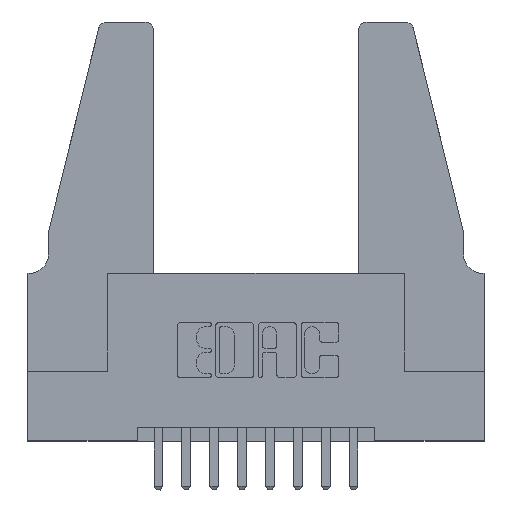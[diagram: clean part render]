
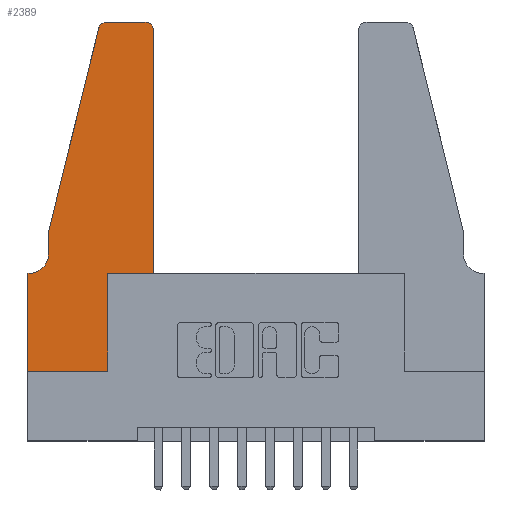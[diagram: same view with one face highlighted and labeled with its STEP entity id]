
A CAD part, top view. The second image highlights one B-rep face of the part: STEP entity #2389.
In plain terms, the highlighted planar face has unit normal (0, 0, 1).
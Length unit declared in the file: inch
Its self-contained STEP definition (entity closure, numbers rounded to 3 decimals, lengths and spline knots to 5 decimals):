
#106 = VECTOR ( 'NONE', #6121, 39.37008 ) ;
#154 = LINE ( 'NONE', #10776, #2517 ) ;
#213 = LINE ( 'NONE', #10357, #3708 ) ;
#300 = CARTESIAN_POINT ( 'NONE',  ( 0.2605, 1.25, 0.37 ) ) ;
#664 = CARTESIAN_POINT ( 'NONE',  ( 0.0755, 0.5, 0.37 ) ) ;
#752 = CARTESIAN_POINT ( 'NONE',  ( 0.4205, 1.25, 0.37 ) ) ;
#1054 = ORIENTED_EDGE ( 'NONE', *, *, #2279, .T. ) ;
#1104 = CARTESIAN_POINT ( 'NONE',  ( 0.4505, 0.35, 0.37 ) ) ;
#1106 = FACE_OUTER_BOUND ( 'NONE', #12802, .T. ) ;
#1151 = ORIENTED_EDGE ( 'NONE', *, *, #7152, .T. ) ;
#1360 = VERTEX_POINT ( 'NONE', #5652 ) ;
#1537 = CARTESIAN_POINT ( 'NONE',  ( 0.4505, 0.35, 0.37 ) ) ;
#1848 = EDGE_CURVE ( 'NONE', #4056, #9533, #4772, .T. ) ;
#1996 = VERTEX_POINT ( 'NONE', #5301 ) ;
#2011 = ORIENTED_EDGE ( 'NONE', *, *, #8331, .T. ) ;
#2022 = CARTESIAN_POINT ( 'NONE',  ( 0.0055, 0.35, 0.37 ) ) ;
#2279 = EDGE_CURVE ( 'NONE', #9148, #5558, #9391, .T. ) ;
#2302 = DIRECTION ( 'NONE',  ( -1., 0., 0. ) ) ;
#2389 = ADVANCED_FACE ( 'NONE', ( #1106 ), #4927, .T. ) ;
#2517 = VECTOR ( 'NONE', #8814, 39.37008 ) ;
#2630 = LINE ( 'NONE', #300, #12486 ) ;
#2672 = VERTEX_POINT ( 'NONE', #1537 ) ;
#2903 = VECTOR ( 'NONE', #11916, 39.37008 ) ;
#3019 = CARTESIAN_POINT ( 'NONE',  ( 0.2865, 0.35, 0.37 ) ) ;
#3112 = ORIENTED_EDGE ( 'NONE', *, *, #9531, .T. ) ;
#3143 = DIRECTION ( 'NONE',  ( 0., 1., 0. ) ) ;
#3332 = VECTOR ( 'NONE', #7789, 39.37008 ) ;
#3708 = VECTOR ( 'NONE', #5157, 39.37008 ) ;
#3750 = LINE ( 'NONE', #1104, #9966 ) ;
#4056 = VERTEX_POINT ( 'NONE', #5022 ) ;
#4112 = DIRECTION ( 'NONE',  ( 0., 0., 1. ) ) ;
#4241 = VERTEX_POINT ( 'NONE', #9990 ) ;
#4388 = CARTESIAN_POINT ( 'NONE',  ( 0.0755, 0.35, 0.37 ) ) ;
#4525 = CARTESIAN_POINT ( 'NONE',  ( 0.284, 1.22, 0.37 ) ) ;
#4729 = VECTOR ( 'NONE', #2302, 39.37008 ) ;
#4732 = CARTESIAN_POINT ( 'NONE',  ( 0.0755, 0.5, 0.37 ) ) ;
#4772 = LINE ( 'NONE', #3019, #6977 ) ;
#4849 = EDGE_CURVE ( 'NONE', #6688, #4056, #9325, .T. ) ;
#4927 = PLANE ( 'NONE',  #9823 ) ;
#5022 = CARTESIAN_POINT ( 'NONE',  ( 0.2865, 0., 0.37 ) ) ;
#5157 = DIRECTION ( 'NONE',  ( 1., 0., 0. ) ) ;
#5158 = EDGE_CURVE ( 'NONE', #1996, #4241, #12277, .T. ) ;
#5301 = CARTESIAN_POINT ( 'NONE',  ( 0.284, 1.25, 0.37 ) ) ;
#5397 = VERTEX_POINT ( 'NONE', #2022 ) ;
#5548 = DIRECTION ( 'NONE',  ( 0., 0., 1. ) ) ;
#5558 = VERTEX_POINT ( 'NONE', #7527 ) ;
#5594 = LINE ( 'NONE', #664, #2903 ) ;
#5596 = DIRECTION ( 'NONE',  ( 1., 0., 0. ) ) ;
#5619 = ORIENTED_EDGE ( 'NONE', *, *, #10081, .T. ) ;
#5630 = VERTEX_POINT ( 'NONE', #7299 ) ;
#5652 = CARTESIAN_POINT ( 'NONE',  ( 0.4505, 1.22, 0.37 ) ) ;
#5856 = ORIENTED_EDGE ( 'NONE', *, *, #10337, .T. ) ;
#5931 = ORIENTED_EDGE ( 'NONE', *, *, #8153, .T. ) ;
#6121 = DIRECTION ( 'NONE',  ( 1., 0., 0. ) ) ;
#6528 = ORIENTED_EDGE ( 'NONE', *, *, #12470, .T. ) ;
#6688 = VERTEX_POINT ( 'NONE', #8548 ) ;
#6740 = ORIENTED_EDGE ( 'NONE', *, *, #4849, .T. ) ;
#6977 = VECTOR ( 'NONE', #12147, 39.37008 ) ;
#6981 = CARTESIAN_POINT ( 'NONE',  ( 0., 0.35, 0.37 ) ) ;
#7152 = EDGE_CURVE ( 'NONE', #1360, #12624, #11939, .T. ) ;
#7299 = CARTESIAN_POINT ( 'NONE',  ( 0., 0.35, 0.37 ) ) ;
#7471 = AXIS2_PLACEMENT_3D ( 'NONE', #12906, #11770, #8734 ) ;
#7527 = CARTESIAN_POINT ( 'NONE',  ( 0.0755, 0.42, 0.37 ) ) ;
#7673 = CARTESIAN_POINT ( 'NONE',  ( 0.4205, 1.22, 0.37 ) ) ;
#7789 = DIRECTION ( 'NONE',  ( 0., -1., 0. ) ) ;
#8053 = ORIENTED_EDGE ( 'NONE', *, *, #1848, .T. ) ;
#8094 = ORIENTED_EDGE ( 'NONE', *, *, #5158, .T. ) ;
#8153 = EDGE_CURVE ( 'NONE', #5630, #6688, #154, .T. ) ;
#8331 = EDGE_CURVE ( 'NONE', #5397, #5630, #12223, .T. ) ;
#8409 = DIRECTION ( 'NONE',  ( -1., 0., 0. ) ) ;
#8548 = CARTESIAN_POINT ( 'NONE',  ( 0., 0., 0.37 ) ) ;
#8677 = DIRECTION ( 'NONE',  ( 1., 0., 0. ) ) ;
#8734 = DIRECTION ( 'NONE',  ( -1., 0., 0. ) ) ;
#8814 = DIRECTION ( 'NONE',  ( 0., -1., 0. ) ) ;
#9148 = VERTEX_POINT ( 'NONE', #11570 ) ;
#9325 = LINE ( 'NONE', #11404, #106 ) ;
#9391 = LINE ( 'NONE', #4732, #3332 ) ;
#9531 = EDGE_CURVE ( 'NONE', #2672, #1360, #3750, .T. ) ;
#9533 = VERTEX_POINT ( 'NONE', #12424 ) ;
#9599 = AXIS2_PLACEMENT_3D ( 'NONE', #4525, #5548, #8677 ) ;
#9823 = AXIS2_PLACEMENT_3D ( 'NONE', #6981, #4112, #12252 ) ;
#9966 = VECTOR ( 'NONE', #3143, 39.37008 ) ;
#9990 = CARTESIAN_POINT ( 'NONE',  ( 0.25487, 1.22718, 0.37 ) ) ;
#10081 = EDGE_CURVE ( 'NONE', #12624, #1996, #2630, .T. ) ;
#10337 = EDGE_CURVE ( 'NONE', #5558, #5397, #11865, .T. ) ;
#10357 = CARTESIAN_POINT ( 'NONE',  ( 0.4505, 0.35, 0.37 ) ) ;
#10776 = CARTESIAN_POINT ( 'NONE',  ( 0., 0., 0.37 ) ) ;
#10785 = DIRECTION ( 'NONE',  ( 0., 0., 1. ) ) ;
#11216 = EDGE_CURVE ( 'NONE', #9533, #2672, #213, .T. ) ;
#11404 = CARTESIAN_POINT ( 'NONE',  ( 0., 0., 0.37 ) ) ;
#11570 = CARTESIAN_POINT ( 'NONE',  ( 0.0755, 0.5, 0.37 ) ) ;
#11770 = DIRECTION ( 'NONE',  ( 0., 0., -1. ) ) ;
#11865 = CIRCLE ( 'NONE', #7471, 0.07 ) ;
#11916 = DIRECTION ( 'NONE',  ( -0.239, -0.971, 0. ) ) ;
#11939 = CIRCLE ( 'NONE', #13004, 0.03 ) ;
#12147 = DIRECTION ( 'NONE',  ( 0., 1., 0. ) ) ;
#12223 = LINE ( 'NONE', #4388, #4729 ) ;
#12252 = DIRECTION ( 'NONE',  ( 1., 0., 0. ) ) ;
#12277 = CIRCLE ( 'NONE', #9599, 0.03 ) ;
#12424 = CARTESIAN_POINT ( 'NONE',  ( 0.2865, 0.35, 0.37 ) ) ;
#12446 = ORIENTED_EDGE ( 'NONE', *, *, #11216, .T. ) ;
#12470 = EDGE_CURVE ( 'NONE', #4241, #9148, #5594, .T. ) ;
#12486 = VECTOR ( 'NONE', #8409, 39.37008 ) ;
#12624 = VERTEX_POINT ( 'NONE', #752 ) ;
#12802 = EDGE_LOOP ( 'NONE', ( #5619, #8094, #6528, #1054, #5856, #2011, #5931, #6740, #8053, #12446, #3112, #1151 ) ) ;
#12906 = CARTESIAN_POINT ( 'NONE',  ( 0.0055, 0.42, 0.37 ) ) ;
#13004 = AXIS2_PLACEMENT_3D ( 'NONE', #7673, #10785, #5596 ) ;
